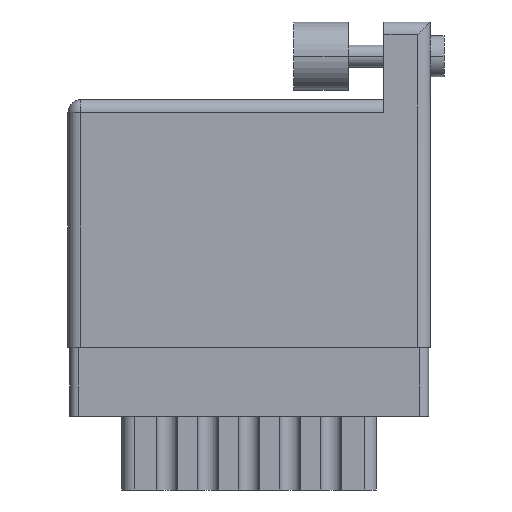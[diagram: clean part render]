
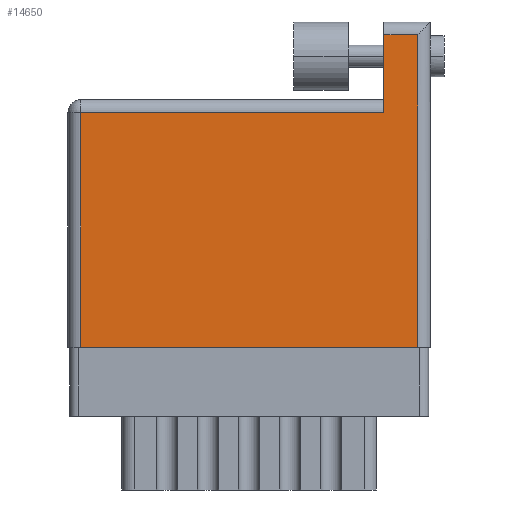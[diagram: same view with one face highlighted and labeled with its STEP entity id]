
A CAD part, front view. The second image highlights one B-rep face of the part: STEP entity #14650.
In plain terms, the highlighted face is planar.
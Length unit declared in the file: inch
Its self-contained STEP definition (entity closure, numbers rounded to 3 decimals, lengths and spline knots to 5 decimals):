
#462 = VERTEX_POINT ( 'NONE', #6077 ) ;
#2096 = ORIENTED_EDGE ( 'NONE', *, *, #3425, .T. ) ;
#2230 = VERTEX_POINT ( 'NONE', #19607 ) ;
#2703 = VERTEX_POINT ( 'NONE', #8392 ) ;
#2952 = CARTESIAN_POINT ( 'NONE',  ( 0.047, 0., 0. ) ) ;
#3228 = CARTESIAN_POINT ( 'NONE',  ( 1.155, 1.143, 0. ) ) ;
#3425 = EDGE_CURVE ( 'NONE', #2230, #11894, #4349, .T. ) ;
#3703 = VECTOR ( 'NONE', #12963, 39.37008 ) ;
#3783 = PLANE ( 'NONE',  #15096 ) ;
#3891 = CARTESIAN_POINT ( 'NONE',  ( 0., 0.906, 0. ) ) ;
#4349 = LINE ( 'NONE', #2952, #14562 ) ;
#4586 = ORIENTED_EDGE ( 'NONE', *, *, #12528, .T. ) ;
#4640 = DIRECTION ( 'NONE',  ( -1., 0., 0. ) ) ;
#4808 = LINE ( 'NONE', #9773, #11614 ) ;
#4931 = CARTESIAN_POINT ( 'NONE',  ( 0.047, 0., 0. ) ) ;
#6077 = CARTESIAN_POINT ( 'NONE',  ( 1.155, 1.143, 0. ) ) ;
#6742 = LINE ( 'NONE', #14707, #18484 ) ;
#6802 = DIRECTION ( 'NONE',  ( 0., 0., -1. ) ) ;
#7935 = ORIENTED_EDGE ( 'NONE', *, *, #12998, .T. ) ;
#8247 = VECTOR ( 'NONE', #4640, 39.37008 ) ;
#8392 = CARTESIAN_POINT ( 'NONE',  ( 1.155, 0.859, 0. ) ) ;
#9773 = CARTESIAN_POINT ( 'NONE',  ( 1.278, 1.19, 0. ) ) ;
#9872 = DIRECTION ( 'NONE',  ( 1., 0., 0. ) ) ;
#10150 = VERTEX_POINT ( 'NONE', #11965 ) ;
#11491 = EDGE_LOOP ( 'NONE', ( #16142, #4586, #19823, #7935, #18266, #2096 ) ) ;
#11536 = EDGE_CURVE ( 'NONE', #2703, #2230, #19064, .T. ) ;
#11555 = LINE ( 'NONE', #21154, #3703 ) ;
#11614 = VECTOR ( 'NONE', #14603, 39.37008 ) ;
#11894 = VERTEX_POINT ( 'NONE', #4931 ) ;
#11965 = CARTESIAN_POINT ( 'NONE',  ( 1.278, 0., 0. ) ) ;
#12528 = EDGE_CURVE ( 'NONE', #10150, #20351, #4808, .T. ) ;
#12588 = EDGE_CURVE ( 'NONE', #11894, #10150, #6742, .T. ) ;
#12948 = VECTOR ( 'NONE', #15414, 39.37008 ) ;
#12963 = DIRECTION ( 'NONE',  ( 0., -1., 0. ) ) ;
#12998 = EDGE_CURVE ( 'NONE', #462, #2703, #11555, .T. ) ;
#14562 = VECTOR ( 'NONE', #18900, 39.37008 ) ;
#14603 = DIRECTION ( 'NONE',  ( 0., 1., 0. ) ) ;
#14650 = ADVANCED_FACE ( 'NONE', ( #18420 ), #3783, .F. ) ;
#14707 = CARTESIAN_POINT ( 'NONE',  ( 0., 0., 0. ) ) ;
#15096 = AXIS2_PLACEMENT_3D ( 'NONE', #3891, #6802, #15311 ) ;
#15311 = DIRECTION ( 'NONE',  ( -1., 0., 0. ) ) ;
#15414 = DIRECTION ( 'NONE',  ( -1., 0., 0. ) ) ;
#16142 = ORIENTED_EDGE ( 'NONE', *, *, #12588, .T. ) ;
#16615 = EDGE_CURVE ( 'NONE', #20351, #462, #19287, .T. ) ;
#18266 = ORIENTED_EDGE ( 'NONE', *, *, #11536, .T. ) ;
#18420 = FACE_OUTER_BOUND ( 'NONE', #11491, .T. ) ;
#18484 = VECTOR ( 'NONE', #9872, 39.37008 ) ;
#18900 = DIRECTION ( 'NONE',  ( 0., -1., 0. ) ) ;
#19064 = LINE ( 'NONE', #20365, #12948 ) ;
#19287 = LINE ( 'NONE', #3228, #8247 ) ;
#19416 = CARTESIAN_POINT ( 'NONE',  ( 1.278, 1.143, 0. ) ) ;
#19607 = CARTESIAN_POINT ( 'NONE',  ( 0.047, 0.859, 0. ) ) ;
#19823 = ORIENTED_EDGE ( 'NONE', *, *, #16615, .T. ) ;
#20351 = VERTEX_POINT ( 'NONE', #19416 ) ;
#20365 = CARTESIAN_POINT ( 'NONE',  ( 0., 0.859, 0. ) ) ;
#21154 = CARTESIAN_POINT ( 'NONE',  ( 1.155, 1.19, 0. ) ) ;
